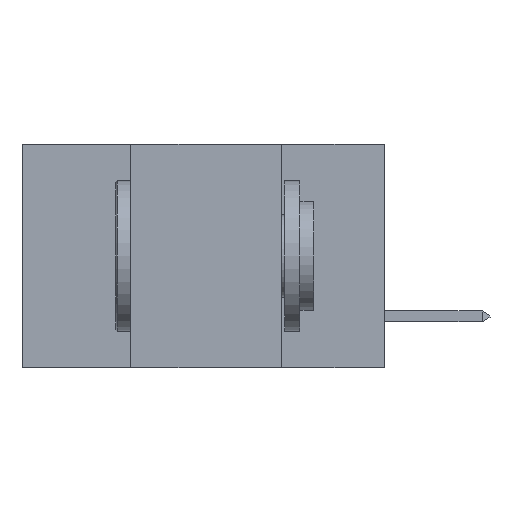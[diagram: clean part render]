
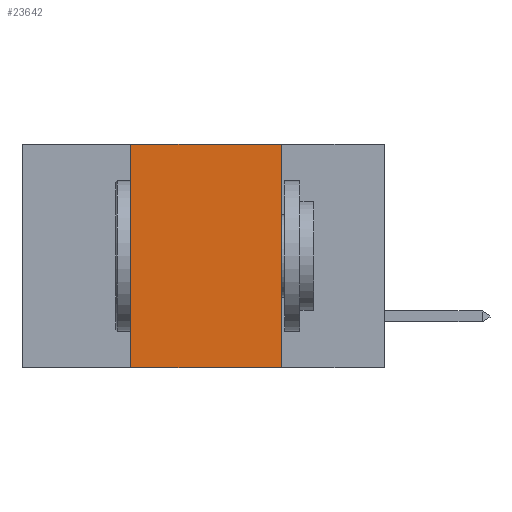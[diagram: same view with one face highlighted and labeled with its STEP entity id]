
A CAD part, left-side view. The second image highlights one B-rep face of the part: STEP entity #23642.
In plain terms, the highlighted planar face has unit normal (-1, 0, 0).
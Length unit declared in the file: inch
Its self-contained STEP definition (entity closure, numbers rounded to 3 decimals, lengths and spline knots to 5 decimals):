
#477 = EDGE_CURVE ( 'NONE', #6263, #3618, #11144, .T. ) ;
#564 = EDGE_CURVE ( 'NONE', #5348, #1037, #25620, .T. ) ;
#1037 = VERTEX_POINT ( 'NONE', #18999 ) ;
#1518 = CARTESIAN_POINT ( 'NONE',  ( 0., 0.6, 0. ) ) ;
#2456 = LINE ( 'NONE', #6595, #13485 ) ;
#3071 = VECTOR ( 'NONE', #20040, 39.37008 ) ;
#3618 = VERTEX_POINT ( 'NONE', #11631 ) ;
#4869 = CARTESIAN_POINT ( 'NONE',  ( 0., 0.6, -0.37 ) ) ;
#5348 = VERTEX_POINT ( 'NONE', #17206 ) ;
#6006 = PLANE ( 'NONE',  #18525 ) ;
#6263 = VERTEX_POINT ( 'NONE', #20648 ) ;
#6595 = CARTESIAN_POINT ( 'NONE',  ( 0., 0.42, 0. ) ) ;
#7054 = CARTESIAN_POINT ( 'NONE',  ( 0., 0.17, 0. ) ) ;
#7420 = EDGE_LOOP ( 'NONE', ( #8980, #17113, #10005, #9312 ) ) ;
#8804 = DIRECTION ( 'NONE',  ( 0., 0., 1. ) ) ;
#8965 = LINE ( 'NONE', #7054, #3071 ) ;
#8980 = ORIENTED_EDGE ( 'NONE', *, *, #17159, .F. ) ;
#9312 = ORIENTED_EDGE ( 'NONE', *, *, #564, .T. ) ;
#10005 = ORIENTED_EDGE ( 'NONE', *, *, #10994, .F. ) ;
#10994 = EDGE_CURVE ( 'NONE', #5348, #6263, #2456, .T. ) ;
#11144 = LINE ( 'NONE', #24410, #16198 ) ;
#11631 = CARTESIAN_POINT ( 'NONE',  ( 0., 0.17, 0. ) ) ;
#12644 = DIRECTION ( 'NONE',  ( 1., 0., 0. ) ) ;
#13485 = VECTOR ( 'NONE', #8804, 39.37008 ) ;
#13808 = FACE_OUTER_BOUND ( 'NONE', #7420, .T. ) ;
#16198 = VECTOR ( 'NONE', #24278, 39.37008 ) ;
#17113 = ORIENTED_EDGE ( 'NONE', *, *, #477, .F. ) ;
#17159 = EDGE_CURVE ( 'NONE', #3618, #1037, #8965, .T. ) ;
#17206 = CARTESIAN_POINT ( 'NONE',  ( 0., 0.42, -0.37 ) ) ;
#17853 = DIRECTION ( 'NONE',  ( 0., -1., 0. ) ) ;
#18525 = AXIS2_PLACEMENT_3D ( 'NONE', #1518, #12644, #27625 ) ;
#18999 = CARTESIAN_POINT ( 'NONE',  ( 0., 0.17, -0.37 ) ) ;
#20040 = DIRECTION ( 'NONE',  ( 0., 0., -1. ) ) ;
#20648 = CARTESIAN_POINT ( 'NONE',  ( 0., 0.42, 0. ) ) ;
#23642 = ADVANCED_FACE ( 'NONE', ( #13808 ), #6006, .F. ) ;
#24278 = DIRECTION ( 'NONE',  ( 0., -1., 0. ) ) ;
#24410 = CARTESIAN_POINT ( 'NONE',  ( 0., 0.6, 0. ) ) ;
#24969 = VECTOR ( 'NONE', #17853, 39.37008 ) ;
#25620 = LINE ( 'NONE', #4869, #24969 ) ;
#27625 = DIRECTION ( 'NONE',  ( 0., 0., -1. ) ) ;
